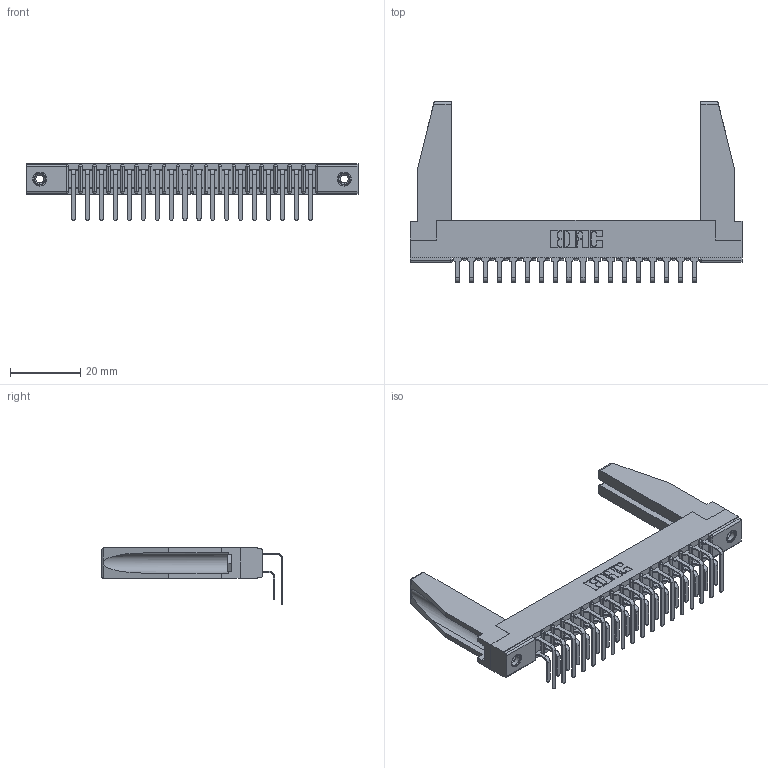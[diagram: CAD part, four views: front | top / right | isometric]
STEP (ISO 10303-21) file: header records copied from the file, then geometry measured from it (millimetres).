
FILE_DESCRIPTION (( 'STEP AP203' ), '1' );
FILE_NAME ('357-018-459-178.STEP', '2020-10-01T00:15:50', ( '' ), ( '' ), 'SwSTEP 2.0', 'SolidWorks 2020', '' );
FILE_SCHEMA (( 'CONFIG_CONTROL_DESIGN' ));
Length unit declared in the file: inch
Products named in the file (6): 307 Part_.156 Dia Mounting Holes; 357-018-459-178; 307-220-078; 345-250-001_345-250-001-102; 307-290-001_558 559 - 1 (Single); 307-290-001_559 - 2 (Single)
Assembly tree (41 placements, depth 2):
  357-018-459-178
    307 Part_.156 Dia Mounting Holes
    307-290-001_558 559 - 1 (Single)  x18
    307-290-001_559 - 2 (Single)  x18
    307-220-078  x2
    345-250-001_345-250-001-102  x2
Bounding box: 94.34 x 51.4 x 16.08 mm (x, y, z)
Volume: 10323.9 mm3; surface area: 15695.3 mm2
Topology: 41 solids, 41 shells, 2067 faces, 5765 edges, 3734 vertices
Faces by surface type: plane 1342, cylinder 671, sphere 38, cone 12, torus 4
Entity records: 22852 total; most frequent: CARTESIAN_POINT 3758, ORIENTED_EDGE 3680, DIRECTION 3644, EDGE_CURVE 1840, LINE 1404, VECTOR 1404, VERTEX_POINT 1192, AXIS2_PLACEMENT_3D 1120
